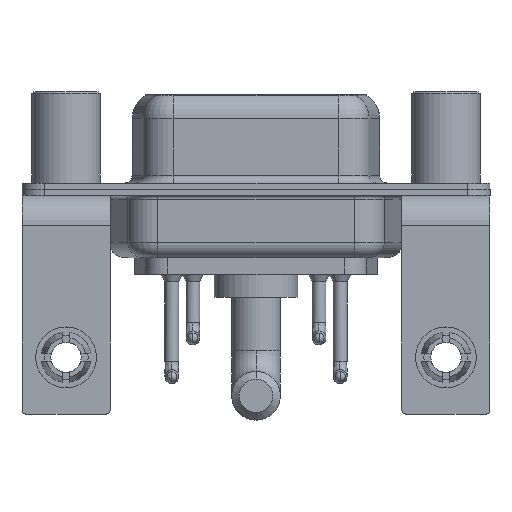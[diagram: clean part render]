
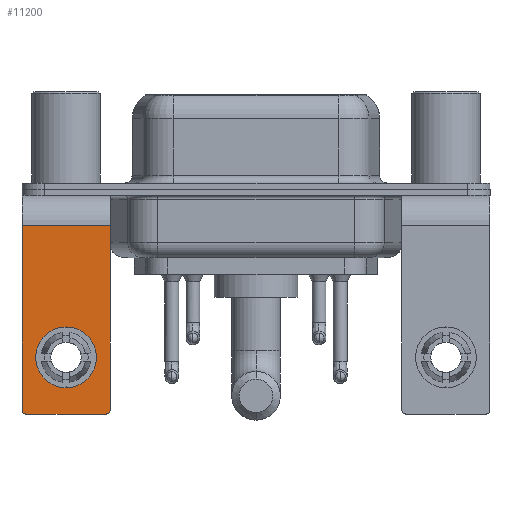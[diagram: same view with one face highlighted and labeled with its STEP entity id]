
A CAD part, front view. The second image highlights one B-rep face of the part: STEP entity #11200.
In plain terms, the highlighted planar face has unit normal (0, -1, 0).
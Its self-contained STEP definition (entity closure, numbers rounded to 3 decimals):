
#110 = CIRCLE ( 'NONE', #10703, 2. ) ;
#365 = CARTESIAN_POINT ( 'NONE',  ( 2.9, -6.25, -2.4 ) ) ;
#704 = ORIENTED_EDGE ( 'NONE', *, *, #17572, .T. ) ;
#723 = DIRECTION ( 'NONE',  ( 0., 1., 0. ) ) ;
#1091 = CARTESIAN_POINT ( 'NONE',  ( -2.9, -6.25, -2.4 ) ) ;
#1162 = AXIS2_PLACEMENT_3D ( 'NONE', #8545, #9993, #3891 ) ;
#1183 = VECTOR ( 'NONE', #12547, 1000. ) ;
#1674 = CARTESIAN_POINT ( 'NONE',  ( -2.9, -6.25, -2.4 ) ) ;
#2275 = CARTESIAN_POINT ( 'NONE',  ( 2.9, -6.25, -2.4 ) ) ;
#2487 = ORIENTED_EDGE ( 'NONE', *, *, #18020, .T. ) ;
#2514 = ORIENTED_EDGE ( 'NONE', *, *, #17249, .F. ) ;
#2545 = CARTESIAN_POINT ( 'NONE',  ( -2.9, -6.25, -14.55 ) ) ;
#3013 = CARTESIAN_POINT ( 'NONE',  ( 0., -6.25, -9.07 ) ) ;
#3053 = AXIS2_PLACEMENT_3D ( 'NONE', #11214, #14308, #17388 ) ;
#3832 = CARTESIAN_POINT ( 'NONE',  ( 2.9, -6.25, -14.55 ) ) ;
#3891 = DIRECTION ( 'NONE',  ( 0., 0., 1. ) ) ;
#4139 = CIRCLE ( 'NONE', #1162, 0.25 ) ;
#4766 = CARTESIAN_POINT ( 'NONE',  ( 2.65, -6.25, -14.8 ) ) ;
#5344 = DIRECTION ( 'NONE',  ( 0., 0., -1. ) ) ;
#5390 = DIRECTION ( 'NONE',  ( 0., 0., 1. ) ) ;
#5880 = EDGE_CURVE ( 'NONE', #11720, #10452, #17369, .T. ) ;
#6095 = CIRCLE ( 'NONE', #3053, 2. ) ;
#6818 = CARTESIAN_POINT ( 'NONE',  ( 2.65, -6.25, -14.55 ) ) ;
#7764 = ORIENTED_EDGE ( 'NONE', *, *, #16408, .F. ) ;
#8545 = CARTESIAN_POINT ( 'NONE',  ( -2.65, -6.25, -14.55 ) ) ;
#8768 = VERTEX_POINT ( 'NONE', #12869 ) ;
#9190 = EDGE_LOOP ( 'NONE', ( #13163, #13704, #7764, #2487, #2514, #17592 ) ) ;
#9722 = EDGE_LOOP ( 'NONE', ( #15932, #704 ) ) ;
#9993 = DIRECTION ( 'NONE',  ( 0., -1., 0. ) ) ;
#10452 = VERTEX_POINT ( 'NONE', #2545 ) ;
#10703 = AXIS2_PLACEMENT_3D ( 'NONE', #19766, #13257, #17893 ) ;
#11034 = VERTEX_POINT ( 'NONE', #4766 ) ;
#11200 = ADVANCED_FACE ( 'NONE', ( #17154, #16431 ), #17667, .F. ) ;
#11213 = LINE ( 'NONE', #14700, #17181 ) ;
#11214 = CARTESIAN_POINT ( 'NONE',  ( 0., -6.25, -11.07 ) ) ;
#11268 = VERTEX_POINT ( 'NONE', #16332 ) ;
#11678 = VERTEX_POINT ( 'NONE', #16306 ) ;
#11720 = VERTEX_POINT ( 'NONE', #1091 ) ;
#12547 = DIRECTION ( 'NONE',  ( 0., 0., -1. ) ) ;
#12656 = DIRECTION ( 'NONE',  ( -1., 0., 0. ) ) ;
#12714 = EDGE_CURVE ( 'NONE', #8768, #11720, #11213, .T. ) ;
#12856 = DIRECTION ( 'NONE',  ( -1., 0., 0. ) ) ;
#12869 = CARTESIAN_POINT ( 'NONE',  ( 2.9, -6.25, -2.4 ) ) ;
#13163 = ORIENTED_EDGE ( 'NONE', *, *, #5880, .T. ) ;
#13257 = DIRECTION ( 'NONE',  ( 0., 1., 0. ) ) ;
#13293 = VECTOR ( 'NONE', #5344, 1000. ) ;
#13704 = ORIENTED_EDGE ( 'NONE', *, *, #20374, .T. ) ;
#14308 = DIRECTION ( 'NONE',  ( 0., 1., 0. ) ) ;
#14700 = CARTESIAN_POINT ( 'NONE',  ( 2.9, -6.25, -2.4 ) ) ;
#15357 = CIRCLE ( 'NONE', #17996, 0.25 ) ;
#15932 = ORIENTED_EDGE ( 'NONE', *, *, #18945, .T. ) ;
#16306 = CARTESIAN_POINT ( 'NONE',  ( 0., -6.25, -13.07 ) ) ;
#16332 = CARTESIAN_POINT ( 'NONE',  ( -2.65, -6.25, -14.8 ) ) ;
#16408 = EDGE_CURVE ( 'NONE', #11034, #11268, #17795, .T. ) ;
#16431 = FACE_OUTER_BOUND ( 'NONE', #9190, .T. ) ;
#16484 = AXIS2_PLACEMENT_3D ( 'NONE', #2275, #723, #5390 ) ;
#16590 = DIRECTION ( 'NONE',  ( 0., 0., 1. ) ) ;
#16698 = DIRECTION ( 'NONE',  ( 0., -1., 0. ) ) ;
#17154 = FACE_BOUND ( 'NONE', #9722, .T. ) ;
#17181 = VECTOR ( 'NONE', #12656, 1000. ) ;
#17249 = EDGE_CURVE ( 'NONE', #8768, #18179, #17925, .T. ) ;
#17369 = LINE ( 'NONE', #1674, #1183 ) ;
#17388 = DIRECTION ( 'NONE',  ( 0., 0., 1. ) ) ;
#17572 = EDGE_CURVE ( 'NONE', #19407, #11678, #6095, .T. ) ;
#17592 = ORIENTED_EDGE ( 'NONE', *, *, #12714, .T. ) ;
#17667 = PLANE ( 'NONE',  #16484 ) ;
#17795 = LINE ( 'NONE', #19565, #19248 ) ;
#17893 = DIRECTION ( 'NONE',  ( 0., 0., 1. ) ) ;
#17925 = LINE ( 'NONE', #365, #13293 ) ;
#17996 = AXIS2_PLACEMENT_3D ( 'NONE', #6818, #16698, #16590 ) ;
#18020 = EDGE_CURVE ( 'NONE', #11034, #18179, #15357, .T. ) ;
#18179 = VERTEX_POINT ( 'NONE', #3832 ) ;
#18945 = EDGE_CURVE ( 'NONE', #11678, #19407, #110, .T. ) ;
#19248 = VECTOR ( 'NONE', #12856, 1000. ) ;
#19407 = VERTEX_POINT ( 'NONE', #3013 ) ;
#19565 = CARTESIAN_POINT ( 'NONE',  ( 2.9, -6.25, -14.8 ) ) ;
#19766 = CARTESIAN_POINT ( 'NONE',  ( 0., -6.25, -11.07 ) ) ;
#20374 = EDGE_CURVE ( 'NONE', #10452, #11268, #4139, .T. ) ;
